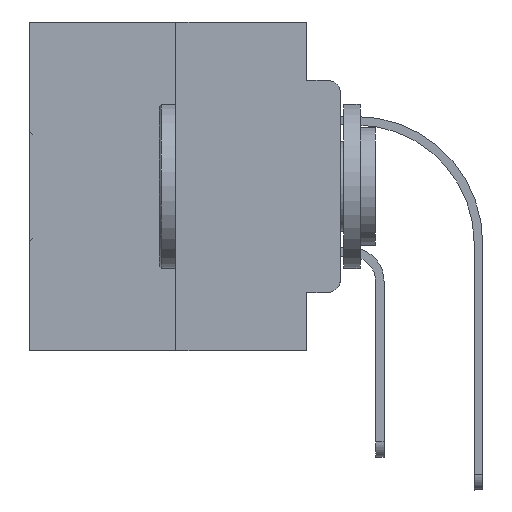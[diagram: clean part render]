
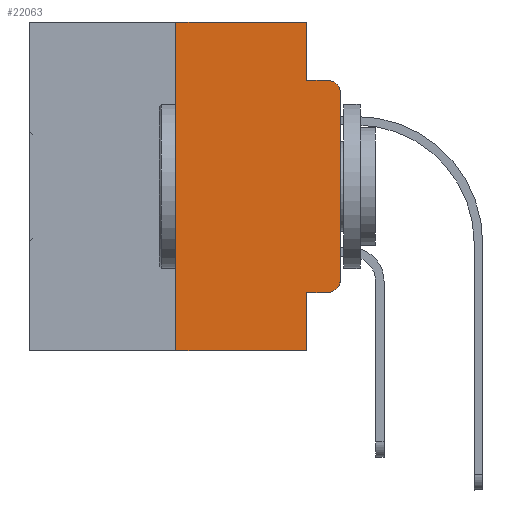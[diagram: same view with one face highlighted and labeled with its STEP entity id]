
A CAD part, left-side view. The second image highlights one B-rep face of the part: STEP entity #22063.
In plain terms, the highlighted planar face has unit normal (-1, 0, 0).
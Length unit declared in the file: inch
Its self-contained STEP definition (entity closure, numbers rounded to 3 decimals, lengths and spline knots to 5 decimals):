
#28 = DIRECTION ( 'NONE',  ( 0., 0., -1. ) ) ;
#809 = EDGE_CURVE ( 'NONE', #30542, #29866, #8092, .T. ) ;
#1164 = VECTOR ( 'NONE', #6201, 39.37008 ) ;
#1996 = CARTESIAN_POINT ( 'NONE',  ( 0., 0.25, 0. ) ) ;
#2308 = LINE ( 'NONE', #15141, #23049 ) ;
#3820 = ORIENTED_EDGE ( 'NONE', *, *, #27436, .T. ) ;
#4086 = CARTESIAN_POINT ( 'NONE',  ( 0., 0.051, 0. ) ) ;
#4113 = ORIENTED_EDGE ( 'NONE', *, *, #12858, .F. ) ;
#4129 = CARTESIAN_POINT ( 'NONE',  ( 0., 0.25, -0.5 ) ) ;
#4609 = DIRECTION ( 'NONE',  ( 0., 0., -1. ) ) ;
#4666 = DIRECTION ( 'NONE',  ( -1., 0., 0. ) ) ;
#5446 = CARTESIAN_POINT ( 'NONE',  ( 0., 0.051, -0.5 ) ) ;
#5458 = VECTOR ( 'NONE', #30177, 39.37008 ) ;
#6201 = DIRECTION ( 'NONE',  ( 0., -1., 0. ) ) ;
#6689 = DIRECTION ( 'NONE',  ( 0., -1., 0. ) ) ;
#7122 = LINE ( 'NONE', #32592, #5458 ) ;
#7205 = CARTESIAN_POINT ( 'NONE',  ( 0., 0., -0.1085 ) ) ;
#7282 = DIRECTION ( 'NONE',  ( 0., -1., 0. ) ) ;
#7340 = DIRECTION ( 'NONE',  ( -1., 0., 0. ) ) ;
#8092 = LINE ( 'NONE', #18512, #24626 ) ;
#9011 = AXIS2_PLACEMENT_3D ( 'NONE', #20498, #7340, #4609 ) ;
#9251 = CARTESIAN_POINT ( 'NONE',  ( 0., 0.02, -0.0885 ) ) ;
#9337 = VECTOR ( 'NONE', #26356, 39.37008 ) ;
#10884 = VECTOR ( 'NONE', #27888, 39.37008 ) ;
#11305 = ORIENTED_EDGE ( 'NONE', *, *, #29292, .F. ) ;
#11654 = LINE ( 'NONE', #21919, #1164 ) ;
#11735 = CIRCLE ( 'NONE', #9011, 0.02 ) ;
#12858 = EDGE_CURVE ( 'NONE', #28008, #21610, #7122, .T. ) ;
#13079 = FACE_OUTER_BOUND ( 'NONE', #18923, .T. ) ;
#13365 = VERTEX_POINT ( 'NONE', #4086 ) ;
#13804 = CARTESIAN_POINT ( 'NONE',  ( 0., 0., 0. ) ) ;
#14434 = VERTEX_POINT ( 'NONE', #7205 ) ;
#14589 = CARTESIAN_POINT ( 'NONE',  ( 0., 0.051, 0. ) ) ;
#15134 = EDGE_CURVE ( 'NONE', #22602, #14434, #24052, .T. ) ;
#15141 = CARTESIAN_POINT ( 'NONE',  ( 0., 0.051, -0.4115 ) ) ;
#15179 = CARTESIAN_POINT ( 'NONE',  ( 0., 0.02, -0.4115 ) ) ;
#15188 = CARTESIAN_POINT ( 'NONE',  ( 0., 0.051, -0.4115 ) ) ;
#15461 = ORIENTED_EDGE ( 'NONE', *, *, #17707, .F. ) ;
#15548 = ORIENTED_EDGE ( 'NONE', *, *, #24319, .T. ) ;
#15831 = CARTESIAN_POINT ( 'NONE',  ( 0., 0.473, 0. ) ) ;
#15950 = CARTESIAN_POINT ( 'NONE',  ( 0., 0.25, 0. ) ) ;
#16202 = CARTESIAN_POINT ( 'NONE',  ( 0., 0.051, -0.0885 ) ) ;
#16281 = EDGE_CURVE ( 'NONE', #18366, #22602, #11735, .T. ) ;
#17680 = CARTESIAN_POINT ( 'NONE',  ( 0., 0., -0.3915 ) ) ;
#17707 = EDGE_CURVE ( 'NONE', #13365, #30542, #25172, .T. ) ;
#18052 = PLANE ( 'NONE',  #24822 ) ;
#18169 = LINE ( 'NONE', #15950, #9337 ) ;
#18366 = VERTEX_POINT ( 'NONE', #15179 ) ;
#18512 = CARTESIAN_POINT ( 'NONE',  ( 0., 0.051, -0.0885 ) ) ;
#18923 = EDGE_LOOP ( 'NONE', ( #24074, #15548, #30327, #15461, #11305, #29934, #3820, #4113, #27292, #23214 ) ) ;
#20034 = LINE ( 'NONE', #33005, #20436 ) ;
#20436 = VECTOR ( 'NONE', #6689, 39.37008 ) ;
#20498 = CARTESIAN_POINT ( 'NONE',  ( 0., 0.02, -0.3915 ) ) ;
#21610 = VERTEX_POINT ( 'NONE', #5446 ) ;
#21919 = CARTESIAN_POINT ( 'NONE',  ( 0., 0.473, 0. ) ) ;
#21980 = AXIS2_PLACEMENT_3D ( 'NONE', #28045, #4666, #28 ) ;
#22063 = ADVANCED_FACE ( 'NONE', ( #13079 ), #18052, .F. ) ;
#22602 = VERTEX_POINT ( 'NONE', #17680 ) ;
#23049 = VECTOR ( 'NONE', #7282, 39.37008 ) ;
#23214 = ORIENTED_EDGE ( 'NONE', *, *, #16281, .T. ) ;
#24052 = LINE ( 'NONE', #13804, #25957 ) ;
#24074 = ORIENTED_EDGE ( 'NONE', *, *, #15134, .T. ) ;
#24223 = DIRECTION ( 'NONE',  ( 0., 0., 1. ) ) ;
#24319 = EDGE_CURVE ( 'NONE', #14434, #29866, #25270, .T. ) ;
#24626 = VECTOR ( 'NONE', #26352, 39.37008 ) ;
#24822 = AXIS2_PLACEMENT_3D ( 'NONE', #15831, #25896, #28621 ) ;
#25172 = LINE ( 'NONE', #14589, #10884 ) ;
#25270 = CIRCLE ( 'NONE', #21980, 0.02 ) ;
#25896 = DIRECTION ( 'NONE',  ( 1., 0., 0. ) ) ;
#25957 = VECTOR ( 'NONE', #24223, 39.37008 ) ;
#26352 = DIRECTION ( 'NONE',  ( 0., -1., 0. ) ) ;
#26356 = DIRECTION ( 'NONE',  ( 0., 0., 1. ) ) ;
#27166 = VERTEX_POINT ( 'NONE', #1996 ) ;
#27292 = ORIENTED_EDGE ( 'NONE', *, *, #30825, .T. ) ;
#27436 = EDGE_CURVE ( 'NONE', #29829, #21610, #20034, .T. ) ;
#27888 = DIRECTION ( 'NONE',  ( 0., 0., -1. ) ) ;
#28008 = VERTEX_POINT ( 'NONE', #15188 ) ;
#28045 = CARTESIAN_POINT ( 'NONE',  ( 0., 0.02, -0.1085 ) ) ;
#28621 = DIRECTION ( 'NONE',  ( 0., 0., -1. ) ) ;
#29152 = EDGE_CURVE ( 'NONE', #29829, #27166, #18169, .T. ) ;
#29292 = EDGE_CURVE ( 'NONE', #27166, #13365, #11654, .T. ) ;
#29829 = VERTEX_POINT ( 'NONE', #4129 ) ;
#29866 = VERTEX_POINT ( 'NONE', #9251 ) ;
#29934 = ORIENTED_EDGE ( 'NONE', *, *, #29152, .F. ) ;
#30177 = DIRECTION ( 'NONE',  ( 0., 0., -1. ) ) ;
#30327 = ORIENTED_EDGE ( 'NONE', *, *, #809, .F. ) ;
#30542 = VERTEX_POINT ( 'NONE', #16202 ) ;
#30825 = EDGE_CURVE ( 'NONE', #28008, #18366, #2308, .T. ) ;
#32592 = CARTESIAN_POINT ( 'NONE',  ( 0., 0.051, 0. ) ) ;
#33005 = CARTESIAN_POINT ( 'NONE',  ( 0., 0.473, -0.5 ) ) ;
